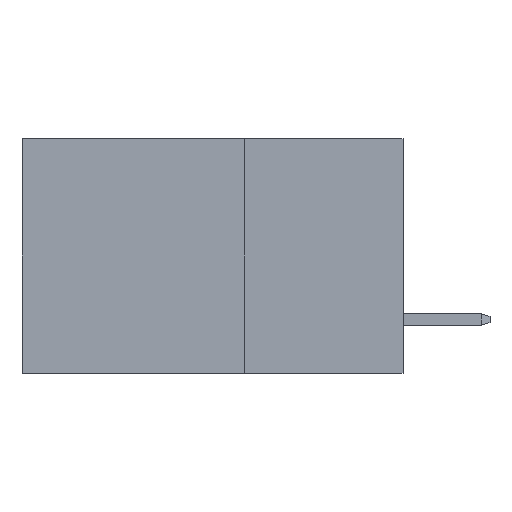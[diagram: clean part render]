
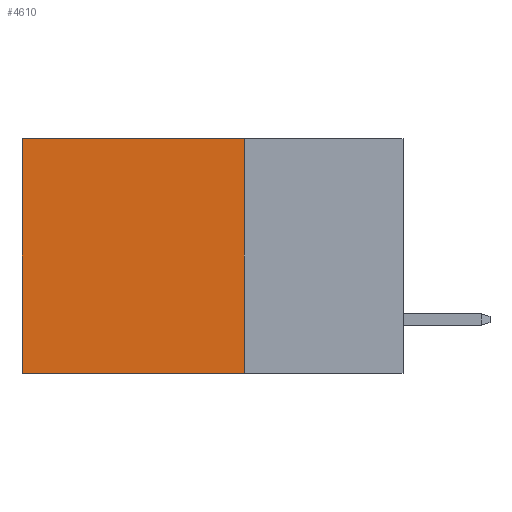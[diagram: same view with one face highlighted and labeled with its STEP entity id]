
A CAD part, left-side view. The second image highlights one B-rep face of the part: STEP entity #4610.
In plain terms, the highlighted planar face has unit normal (-1, 0, 0).
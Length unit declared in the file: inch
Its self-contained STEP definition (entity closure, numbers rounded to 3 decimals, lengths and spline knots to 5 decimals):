
#287 = PLANE ( 'NONE',  #5210 ) ;
#547 = VECTOR ( 'NONE', #2335, 39.37008 ) ;
#957 = CARTESIAN_POINT ( 'NONE',  ( 0.2875, 0.25, 0. ) ) ;
#1081 = FACE_OUTER_BOUND ( 'NONE', #5734, .T. ) ;
#1266 = CARTESIAN_POINT ( 'NONE',  ( 0.2875, 0.25, -0.37 ) ) ;
#1648 = LINE ( 'NONE', #3618, #1960 ) ;
#1960 = VECTOR ( 'NONE', #5655, 39.37008 ) ;
#2115 = CARTESIAN_POINT ( 'NONE',  ( 0.2875, 0.25, 0. ) ) ;
#2250 = LINE ( 'NONE', #7649, #5111 ) ;
#2335 = DIRECTION ( 'NONE',  ( 0., 0., -1. ) ) ;
#2967 = CARTESIAN_POINT ( 'NONE',  ( 0.2875, 0.6, -0.37 ) ) ;
#3010 = CARTESIAN_POINT ( 'NONE',  ( 0.2875, 0.6, 0. ) ) ;
#3618 = CARTESIAN_POINT ( 'NONE',  ( 0.2875, 0.25, -0.37 ) ) ;
#3703 = ORIENTED_EDGE ( 'NONE', *, *, #8559, .F. ) ;
#3704 = ORIENTED_EDGE ( 'NONE', *, *, #8454, .T. ) ;
#4392 = VERTEX_POINT ( 'NONE', #1266 ) ;
#4522 = ORIENTED_EDGE ( 'NONE', *, *, #8833, .F. ) ;
#4610 = ADVANCED_FACE ( 'NONE', ( #1081 ), #287, .F. ) ;
#4823 = VECTOR ( 'NONE', #8370, 39.37008 ) ;
#5017 = DIRECTION ( 'NONE',  ( 1., 0., 0. ) ) ;
#5111 = VECTOR ( 'NONE', #7694, 39.37008 ) ;
#5210 = AXIS2_PLACEMENT_3D ( 'NONE', #957, #5017, #5310 ) ;
#5310 = DIRECTION ( 'NONE',  ( 0., 0., -1. ) ) ;
#5456 = LINE ( 'NONE', #2115, #4823 ) ;
#5655 = DIRECTION ( 'NONE',  ( 0., 1., 0. ) ) ;
#5734 = EDGE_LOOP ( 'NONE', ( #8768, #4522, #3703, #3704 ) ) ;
#6076 = VERTEX_POINT ( 'NONE', #3010 ) ;
#7100 = VERTEX_POINT ( 'NONE', #2967 ) ;
#7350 = CARTESIAN_POINT ( 'NONE',  ( 0.2875, 0.6, 0. ) ) ;
#7649 = CARTESIAN_POINT ( 'NONE',  ( 0.2875, 0.25, 0. ) ) ;
#7694 = DIRECTION ( 'NONE',  ( 0., 0., -1. ) ) ;
#8031 = VERTEX_POINT ( 'NONE', #8730 ) ;
#8370 = DIRECTION ( 'NONE',  ( 0., 1., 0. ) ) ;
#8454 = EDGE_CURVE ( 'NONE', #8031, #6076, #5456, .T. ) ;
#8559 = EDGE_CURVE ( 'NONE', #8031, #4392, #2250, .T. ) ;
#8616 = LINE ( 'NONE', #7350, #547 ) ;
#8698 = EDGE_CURVE ( 'NONE', #6076, #7100, #8616, .T. ) ;
#8730 = CARTESIAN_POINT ( 'NONE',  ( 0.2875, 0.25, 0. ) ) ;
#8768 = ORIENTED_EDGE ( 'NONE', *, *, #8698, .T. ) ;
#8833 = EDGE_CURVE ( 'NONE', #4392, #7100, #1648, .T. ) ;
